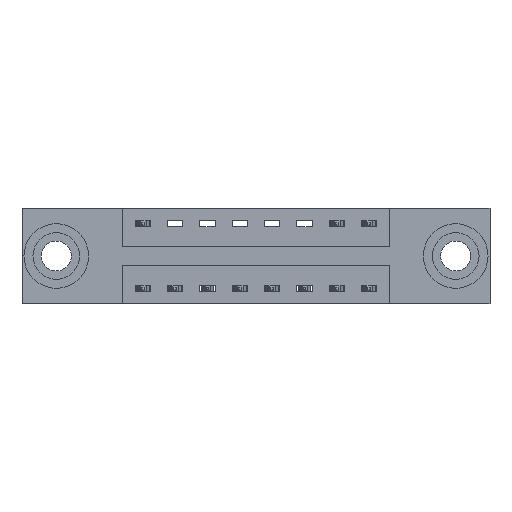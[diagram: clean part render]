
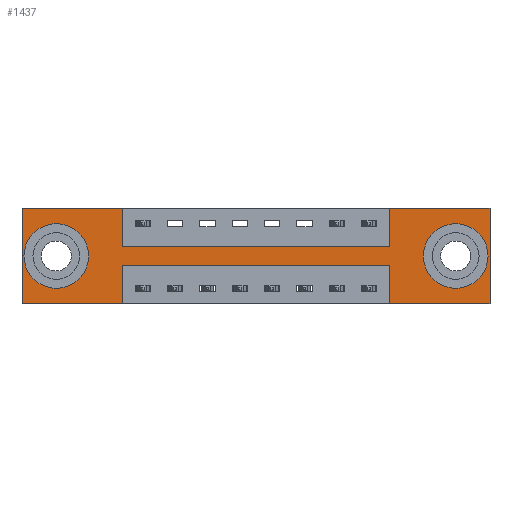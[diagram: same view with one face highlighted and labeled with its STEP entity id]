
A CAD part, front view. The second image highlights one B-rep face of the part: STEP entity #1437.
In plain terms, the highlighted planar face has unit normal (0, -1, 0).
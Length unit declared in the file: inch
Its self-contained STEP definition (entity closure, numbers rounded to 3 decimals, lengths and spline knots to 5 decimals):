
#7 = ORIENTED_EDGE ( 'NONE', *, *, #4065, .F. ) ;
#20 = ORIENTED_EDGE ( 'NONE', *, *, #7100, .F. ) ;
#32 = EDGE_LOOP ( 'NONE', ( #5815, #5840, #5859, #5905, #2597, #7, #20, #114, #152, #249, #339, #343 ) ) ;
#114 = ORIENTED_EDGE ( 'NONE', *, *, #4821, .F. ) ;
#152 = ORIENTED_EDGE ( 'NONE', *, *, #4955, .F. ) ;
#249 = ORIENTED_EDGE ( 'NONE', *, *, #6921, .F. ) ;
#339 = ORIENTED_EDGE ( 'NONE', *, *, #5520, .F. ) ;
#343 = ORIENTED_EDGE ( 'NONE', *, *, #5479, .F. ) ;
#402 = LINE ( 'NONE', #2588, #2130 ) ;
#471 = CARTESIAN_POINT ( 'NONE',  ( 0.3875, 0., -0.22 ) ) ;
#477 = VERTEX_POINT ( 'NONE', #9525 ) ;
#591 = EDGE_CURVE ( 'NONE', #8837, #477, #5120, .T. ) ;
#626 = DIRECTION ( 'NONE',  ( 1., 0., 0. ) ) ;
#688 = DIRECTION ( 'NONE',  ( 0., 0., 1. ) ) ;
#721 = CARTESIAN_POINT ( 'NONE',  ( 1.4225, 0., -0.37 ) ) ;
#770 = DIRECTION ( 'NONE',  ( -1., 0., 0. ) ) ;
#1004 = EDGE_CURVE ( 'NONE', #1296, #3185, #9233, .T. ) ;
#1028 = LINE ( 'NONE', #10328, #5318 ) ;
#1176 = CARTESIAN_POINT ( 'NONE',  ( 1.4225, 0., -0.37 ) ) ;
#1214 = AXIS2_PLACEMENT_3D ( 'NONE', #7077, #3260, #4861 ) ;
#1264 = EDGE_LOOP ( 'NONE', ( #6213, #5585 ) ) ;
#1283 = VECTOR ( 'NONE', #5018, 39.37008 ) ;
#1296 = VERTEX_POINT ( 'NONE', #5428 ) ;
#1306 = DIRECTION ( 'NONE',  ( 1., 0., 0. ) ) ;
#1380 = VERTEX_POINT ( 'NONE', #2641 ) ;
#1437 = ADVANCED_FACE ( 'NONE', ( #8769, #8993, #2823 ), #3850, .T. ) ;
#1523 = VERTEX_POINT ( 'NONE', #1176 ) ;
#1547 = DIRECTION ( 'NONE',  ( 0., 0., -1. ) ) ;
#1599 = CARTESIAN_POINT ( 'NONE',  ( 0.3875, 0., -0.37 ) ) ;
#1632 = VERTEX_POINT ( 'NONE', #10050 ) ;
#1823 = CARTESIAN_POINT ( 'NONE',  ( 1.4225, 0., -0.22 ) ) ;
#2130 = VECTOR ( 'NONE', #2572, 39.37008 ) ;
#2255 = DIRECTION ( 'NONE',  ( -1., 0., 0. ) ) ;
#2280 = VERTEX_POINT ( 'NONE', #1823 ) ;
#2300 = EDGE_CURVE ( 'NONE', #2375, #6405, #5967, .T. ) ;
#2375 = VERTEX_POINT ( 'NONE', #471 ) ;
#2541 = DIRECTION ( 'NONE',  ( 0., 0., 1. ) ) ;
#2572 = DIRECTION ( 'NONE',  ( 1., 0., 0. ) ) ;
#2588 = CARTESIAN_POINT ( 'NONE',  ( 0., 0., 0. ) ) ;
#2597 = ORIENTED_EDGE ( 'NONE', *, *, #2764, .F. ) ;
#2641 = CARTESIAN_POINT ( 'NONE',  ( 1.81, 0., 0. ) ) ;
#2764 = EDGE_CURVE ( 'NONE', #1380, #7498, #7192, .T. ) ;
#2823 = FACE_OUTER_BOUND ( 'NONE', #32, .T. ) ;
#2920 = VECTOR ( 'NONE', #1306, 39.37008 ) ;
#2967 = CARTESIAN_POINT ( 'NONE',  ( 1.4225, 0., 0. ) ) ;
#2985 = DIRECTION ( 'NONE',  ( 0., 0., 1. ) ) ;
#2996 = DIRECTION ( 'NONE',  ( 0., 1., 0. ) ) ;
#3029 = CARTESIAN_POINT ( 'NONE',  ( 0.1325, 0., -0.185 ) ) ;
#3185 = VERTEX_POINT ( 'NONE', #6547 ) ;
#3260 = DIRECTION ( 'NONE',  ( 0., 1., 0. ) ) ;
#3403 = CARTESIAN_POINT ( 'NONE',  ( 0., 0., -0.37 ) ) ;
#3560 = CARTESIAN_POINT ( 'NONE',  ( 0., 0., -0.37 ) ) ;
#3619 = CARTESIAN_POINT ( 'NONE',  ( 1.6775, 0., -0.185 ) ) ;
#3844 = DIRECTION ( 'NONE',  ( 0., 0., -1. ) ) ;
#3850 = PLANE ( 'NONE',  #9516 ) ;
#3896 = VERTEX_POINT ( 'NONE', #3560 ) ;
#3974 = EDGE_CURVE ( 'NONE', #477, #8837, #9742, .T. ) ;
#3976 = CARTESIAN_POINT ( 'NONE',  ( 0.3875, 0., -0.37 ) ) ;
#3978 = VERTEX_POINT ( 'NONE', #2967 ) ;
#4036 = CARTESIAN_POINT ( 'NONE',  ( 0., 0., 0. ) ) ;
#4065 = EDGE_CURVE ( 'NONE', #3978, #1380, #402, .T. ) ;
#4166 = CARTESIAN_POINT ( 'NONE',  ( 0.3875, 0., 0. ) ) ;
#4408 = EDGE_CURVE ( 'NONE', #1523, #2280, #9085, .T. ) ;
#4497 = AXIS2_PLACEMENT_3D ( 'NONE', #3619, #7259, #3844 ) ;
#4770 = CARTESIAN_POINT ( 'NONE',  ( 0.3875, 0., -0.15 ) ) ;
#4821 = EDGE_CURVE ( 'NONE', #6415, #8600, #5440, .T. ) ;
#4861 = DIRECTION ( 'NONE',  ( 0., 0., 1. ) ) ;
#4929 = CARTESIAN_POINT ( 'NONE',  ( 1.6775, 0., -0.185 ) ) ;
#4955 = EDGE_CURVE ( 'NONE', #1632, #6415, #5831, .T. ) ;
#4987 = EDGE_CURVE ( 'NONE', #7498, #1523, #1028, .T. ) ;
#5018 = DIRECTION ( 'NONE',  ( 0., 0., -1. ) ) ;
#5092 = VECTOR ( 'NONE', #8451, 39.37008 ) ;
#5120 = CIRCLE ( 'NONE', #1214, 0.078 ) ;
#5171 = VECTOR ( 'NONE', #2541, 39.37008 ) ;
#5314 = DIRECTION ( 'NONE',  ( 0., 0., 1. ) ) ;
#5318 = VECTOR ( 'NONE', #770, 39.37008 ) ;
#5399 = AXIS2_PLACEMENT_3D ( 'NONE', #3029, #2996, #2985 ) ;
#5428 = CARTESIAN_POINT ( 'NONE',  ( 1.6775, 0., -0.263 ) ) ;
#5440 = LINE ( 'NONE', #4770, #2920 ) ;
#5479 = EDGE_CURVE ( 'NONE', #6405, #3896, #9731, .T. ) ;
#5520 = EDGE_CURVE ( 'NONE', #3896, #7561, #9522, .T. ) ;
#5585 = ORIENTED_EDGE ( 'NONE', *, *, #1004, .T. ) ;
#5639 = CARTESIAN_POINT ( 'NONE',  ( 0.1325, 0., -0.107 ) ) ;
#5724 = ORIENTED_EDGE ( 'NONE', *, *, #591, .T. ) ;
#5731 = DIRECTION ( 'NONE',  ( 0., 0., -1. ) ) ;
#5739 = ORIENTED_EDGE ( 'NONE', *, *, #3974, .T. ) ;
#5815 = ORIENTED_EDGE ( 'NONE', *, *, #2300, .F. ) ;
#5831 = LINE ( 'NONE', #4166, #1283 ) ;
#5840 = ORIENTED_EDGE ( 'NONE', *, *, #6838, .F. ) ;
#5859 = ORIENTED_EDGE ( 'NONE', *, *, #4408, .F. ) ;
#5905 = ORIENTED_EDGE ( 'NONE', *, *, #4987, .F. ) ;
#5924 = EDGE_CURVE ( 'NONE', #3185, #1296, #6789, .T. ) ;
#5967 = LINE ( 'NONE', #1599, #7796 ) ;
#6213 = ORIENTED_EDGE ( 'NONE', *, *, #5924, .T. ) ;
#6391 = LINE ( 'NONE', #8001, #8452 ) ;
#6405 = VERTEX_POINT ( 'NONE', #3976 ) ;
#6415 = VERTEX_POINT ( 'NONE', #6441 ) ;
#6441 = CARTESIAN_POINT ( 'NONE',  ( 0.3875, 0., -0.15 ) ) ;
#6547 = CARTESIAN_POINT ( 'NONE',  ( 1.6775, 0., -0.107 ) ) ;
#6756 = VECTOR ( 'NONE', #5314, 39.37008 ) ;
#6789 = CIRCLE ( 'NONE', #7341, 0.078 ) ;
#6838 = EDGE_CURVE ( 'NONE', #2280, #2375, #6391, .T. ) ;
#6921 = EDGE_CURVE ( 'NONE', #7561, #1632, #10130, .T. ) ;
#7068 = VECTOR ( 'NONE', #688, 39.37008 ) ;
#7077 = CARTESIAN_POINT ( 'NONE',  ( 0.1325, 0., -0.185 ) ) ;
#7100 = EDGE_CURVE ( 'NONE', #8600, #3978, #9020, .T. ) ;
#7192 = LINE ( 'NONE', #8630, #5092 ) ;
#7259 = DIRECTION ( 'NONE',  ( 0., 1., 0. ) ) ;
#7278 = CARTESIAN_POINT ( 'NONE',  ( 0., 0., 0. ) ) ;
#7341 = AXIS2_PLACEMENT_3D ( 'NONE', #4929, #10220, #5731 ) ;
#7445 = DIRECTION ( 'NONE',  ( -1., 0., 0. ) ) ;
#7498 = VERTEX_POINT ( 'NONE', #9458 ) ;
#7561 = VERTEX_POINT ( 'NONE', #4036 ) ;
#7770 = VECTOR ( 'NONE', #7445, 39.37008 ) ;
#7796 = VECTOR ( 'NONE', #1547, 39.37008 ) ;
#8001 = CARTESIAN_POINT ( 'NONE',  ( 0.3875, 0., -0.22 ) ) ;
#8175 = EDGE_LOOP ( 'NONE', ( #5724, #5739 ) ) ;
#8272 = CARTESIAN_POINT ( 'NONE',  ( 0., 0., 0. ) ) ;
#8285 = DIRECTION ( 'NONE',  ( 0., -1., 0. ) ) ;
#8429 = CARTESIAN_POINT ( 'NONE',  ( 1.4225, 0., 0. ) ) ;
#8451 = DIRECTION ( 'NONE',  ( 0., 0., -1. ) ) ;
#8452 = VECTOR ( 'NONE', #2255, 39.37008 ) ;
#8600 = VERTEX_POINT ( 'NONE', #9955 ) ;
#8630 = CARTESIAN_POINT ( 'NONE',  ( 1.81, 0., 0. ) ) ;
#8769 = FACE_BOUND ( 'NONE', #1264, .T. ) ;
#8837 = VERTEX_POINT ( 'NONE', #5639 ) ;
#8993 = FACE_BOUND ( 'NONE', #8175, .T. ) ;
#9020 = LINE ( 'NONE', #8429, #6756 ) ;
#9085 = LINE ( 'NONE', #721, #7068 ) ;
#9233 = CIRCLE ( 'NONE', #4497, 0.078 ) ;
#9458 = CARTESIAN_POINT ( 'NONE',  ( 1.81, 0., -0.37 ) ) ;
#9516 = AXIS2_PLACEMENT_3D ( 'NONE', #3403, #8285, #9968 ) ;
#9522 = LINE ( 'NONE', #8272, #5171 ) ;
#9525 = CARTESIAN_POINT ( 'NONE',  ( 0.1325, 0., -0.263 ) ) ;
#9662 = CARTESIAN_POINT ( 'NONE',  ( 0., 0., -0.37 ) ) ;
#9731 = LINE ( 'NONE', #9662, #7770 ) ;
#9742 = CIRCLE ( 'NONE', #5399, 0.078 ) ;
#9920 = VECTOR ( 'NONE', #626, 39.37008 ) ;
#9955 = CARTESIAN_POINT ( 'NONE',  ( 1.4225, 0., -0.15 ) ) ;
#9968 = DIRECTION ( 'NONE',  ( 0., 0., -1. ) ) ;
#10050 = CARTESIAN_POINT ( 'NONE',  ( 0.3875, 0., 0. ) ) ;
#10130 = LINE ( 'NONE', #7278, #9920 ) ;
#10220 = DIRECTION ( 'NONE',  ( 0., 1., 0. ) ) ;
#10328 = CARTESIAN_POINT ( 'NONE',  ( 0., 0., -0.37 ) ) ;
